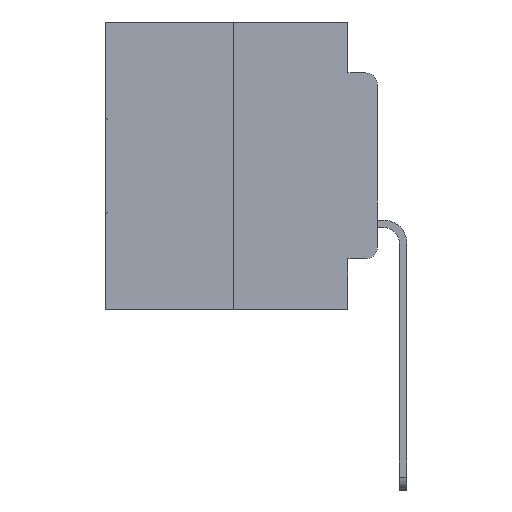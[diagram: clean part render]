
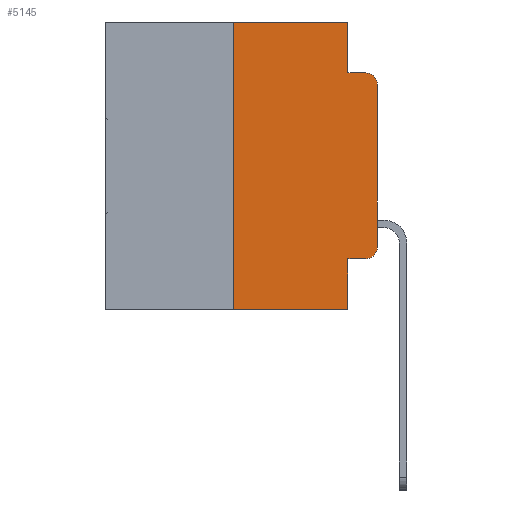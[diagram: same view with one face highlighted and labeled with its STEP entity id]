
A CAD part, left-side view. The second image highlights one B-rep face of the part: STEP entity #5145.
In plain terms, the highlighted planar face has unit normal (-1, 0, 0).
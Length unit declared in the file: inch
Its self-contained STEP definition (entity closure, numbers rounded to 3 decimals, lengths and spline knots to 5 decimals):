
#289 = CARTESIAN_POINT ( 'NONE',  ( 0., 0.473, 0. ) ) ;
#721 = DIRECTION ( 'NONE',  ( 0., -1., 0. ) ) ;
#1280 = AXIS2_PLACEMENT_3D ( 'NONE', #18541, #4584, #20802 ) ;
#1391 = EDGE_CURVE ( 'NONE', #30093, #17878, #15419, .T. ) ;
#2750 = DIRECTION ( 'NONE',  ( 0., -1., 0. ) ) ;
#3092 = PLANE ( 'NONE',  #4730 ) ;
#3249 = CARTESIAN_POINT ( 'NONE',  ( 0., 0.02, -0.3915 ) ) ;
#3373 = LINE ( 'NONE', #12487, #15217 ) ;
#3385 = VECTOR ( 'NONE', #6405, 39.37008 ) ;
#3609 = VERTEX_POINT ( 'NONE', #27569 ) ;
#3971 = CARTESIAN_POINT ( 'NONE',  ( 0., 0.051, -0.4115 ) ) ;
#4584 = DIRECTION ( 'NONE',  ( -1., 0., 0. ) ) ;
#4730 = AXIS2_PLACEMENT_3D ( 'NONE', #6817, #12664, #13833 ) ;
#5145 = ADVANCED_FACE ( 'NONE', ( #13674 ), #3092, .F. ) ;
#5207 = ORIENTED_EDGE ( 'NONE', *, *, #18217, .F. ) ;
#5748 = DIRECTION ( 'NONE',  ( 0., 0., -1. ) ) ;
#6405 = DIRECTION ( 'NONE',  ( 0., -1., 0. ) ) ;
#6425 = VERTEX_POINT ( 'NONE', #15278 ) ;
#6817 = CARTESIAN_POINT ( 'NONE',  ( 0., 0.473, 0. ) ) ;
#6819 = AXIS2_PLACEMENT_3D ( 'NONE', #3249, #19637, #5748 ) ;
#7144 = EDGE_LOOP ( 'NONE', ( #13299, #17268, #15526, #8515, #5207, #20266, #24704, #22946, #22686, #16637 ) ) ;
#7700 = VERTEX_POINT ( 'NONE', #25110 ) ;
#7925 = CIRCLE ( 'NONE', #1280, 0.02 ) ;
#8356 = EDGE_CURVE ( 'NONE', #3609, #17878, #19117, .T. ) ;
#8433 = CARTESIAN_POINT ( 'NONE',  ( 0., 0.051, 0. ) ) ;
#8515 = ORIENTED_EDGE ( 'NONE', *, *, #12089, .F. ) ;
#8529 = LINE ( 'NONE', #289, #26932 ) ;
#8573 = VERTEX_POINT ( 'NONE', #29851 ) ;
#8972 = CARTESIAN_POINT ( 'NONE',  ( 0., 0.051, 0. ) ) ;
#9618 = CARTESIAN_POINT ( 'NONE',  ( 0., 0.02, -0.0885 ) ) ;
#10061 = EDGE_CURVE ( 'NONE', #8573, #11736, #23330, .T. ) ;
#11074 = CARTESIAN_POINT ( 'NONE',  ( 0., 0.051, -0.5 ) ) ;
#11736 = VERTEX_POINT ( 'NONE', #9618 ) ;
#12089 = EDGE_CURVE ( 'NONE', #22125, #8573, #3373, .T. ) ;
#12147 = EDGE_CURVE ( 'NONE', #12327, #6425, #25979, .T. ) ;
#12327 = VERTEX_POINT ( 'NONE', #27564 ) ;
#12350 = DIRECTION ( 'NONE',  ( 0., 0., 1. ) ) ;
#12363 = EDGE_CURVE ( 'NONE', #7700, #11736, #7925, .T. ) ;
#12487 = CARTESIAN_POINT ( 'NONE',  ( 0., 0.051, 0. ) ) ;
#12664 = DIRECTION ( 'NONE',  ( 1., 0., 0. ) ) ;
#12746 = CARTESIAN_POINT ( 'NONE',  ( 0., 0.051, -0.0885 ) ) ;
#13299 = ORIENTED_EDGE ( 'NONE', *, *, #19238, .T. ) ;
#13674 = FACE_OUTER_BOUND ( 'NONE', #7144, .T. ) ;
#13817 = VECTOR ( 'NONE', #23438, 39.37008 ) ;
#13833 = DIRECTION ( 'NONE',  ( 0., 0., -1. ) ) ;
#14232 = EDGE_CURVE ( 'NONE', #3609, #21204, #23526, .T. ) ;
#14405 = CARTESIAN_POINT ( 'NONE',  ( 0., 0.051, -0.4115 ) ) ;
#14794 = DIRECTION ( 'NONE',  ( 0., 0., -1. ) ) ;
#15217 = VECTOR ( 'NONE', #14794, 39.37008 ) ;
#15278 = CARTESIAN_POINT ( 'NONE',  ( 0., 0., -0.3915 ) ) ;
#15419 = LINE ( 'NONE', #8972, #20739 ) ;
#15526 = ORIENTED_EDGE ( 'NONE', *, *, #10061, .F. ) ;
#16282 = DIRECTION ( 'NONE',  ( 0., 0., -1. ) ) ;
#16637 = ORIENTED_EDGE ( 'NONE', *, *, #12147, .T. ) ;
#17268 = ORIENTED_EDGE ( 'NONE', *, *, #12363, .T. ) ;
#17269 = VECTOR ( 'NONE', #721, 39.37008 ) ;
#17878 = VERTEX_POINT ( 'NONE', #11074 ) ;
#18217 = EDGE_CURVE ( 'NONE', #21204, #22125, #8529, .T. ) ;
#18541 = CARTESIAN_POINT ( 'NONE',  ( 0., 0.02, -0.1085 ) ) ;
#18672 = DIRECTION ( 'NONE',  ( 0., 0., 1. ) ) ;
#19038 = CARTESIAN_POINT ( 'NONE',  ( 0., 0.25, 0. ) ) ;
#19098 = CARTESIAN_POINT ( 'NONE',  ( 0., 0., 0. ) ) ;
#19117 = LINE ( 'NONE', #21081, #13817 ) ;
#19238 = EDGE_CURVE ( 'NONE', #6425, #7700, #27217, .T. ) ;
#19637 = DIRECTION ( 'NONE',  ( -1., 0., 0. ) ) ;
#20266 = ORIENTED_EDGE ( 'NONE', *, *, #14232, .F. ) ;
#20739 = VECTOR ( 'NONE', #16282, 39.37008 ) ;
#20802 = DIRECTION ( 'NONE',  ( 0., 0., -1. ) ) ;
#21068 = VECTOR ( 'NONE', #12350, 39.37008 ) ;
#21081 = CARTESIAN_POINT ( 'NONE',  ( 0., 0.473, -0.5 ) ) ;
#21204 = VERTEX_POINT ( 'NONE', #19038 ) ;
#22001 = LINE ( 'NONE', #3971, #3385 ) ;
#22125 = VERTEX_POINT ( 'NONE', #8433 ) ;
#22686 = ORIENTED_EDGE ( 'NONE', *, *, #24379, .T. ) ;
#22946 = ORIENTED_EDGE ( 'NONE', *, *, #1391, .F. ) ;
#23330 = LINE ( 'NONE', #12746, #17269 ) ;
#23438 = DIRECTION ( 'NONE',  ( 0., -1., 0. ) ) ;
#23526 = LINE ( 'NONE', #25510, #28796 ) ;
#24379 = EDGE_CURVE ( 'NONE', #30093, #12327, #22001, .T. ) ;
#24704 = ORIENTED_EDGE ( 'NONE', *, *, #8356, .T. ) ;
#25110 = CARTESIAN_POINT ( 'NONE',  ( 0., 0., -0.1085 ) ) ;
#25510 = CARTESIAN_POINT ( 'NONE',  ( 0., 0.25, 0. ) ) ;
#25979 = CIRCLE ( 'NONE', #6819, 0.02 ) ;
#26932 = VECTOR ( 'NONE', #2750, 39.37008 ) ;
#27217 = LINE ( 'NONE', #19098, #21068 ) ;
#27564 = CARTESIAN_POINT ( 'NONE',  ( 0., 0.02, -0.4115 ) ) ;
#27569 = CARTESIAN_POINT ( 'NONE',  ( 0., 0.25, -0.5 ) ) ;
#28796 = VECTOR ( 'NONE', #18672, 39.37008 ) ;
#29851 = CARTESIAN_POINT ( 'NONE',  ( 0., 0.051, -0.0885 ) ) ;
#30093 = VERTEX_POINT ( 'NONE', #14405 ) ;
